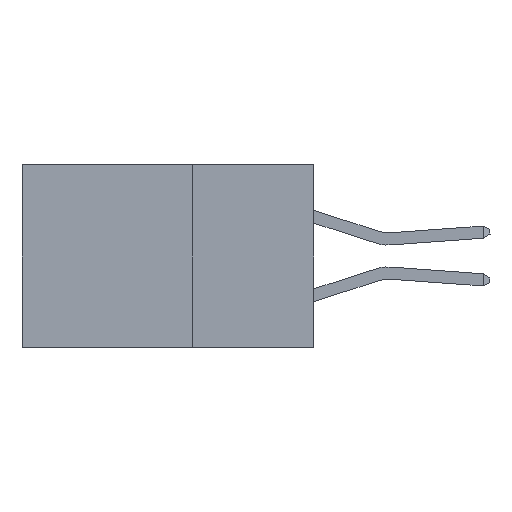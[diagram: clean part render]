
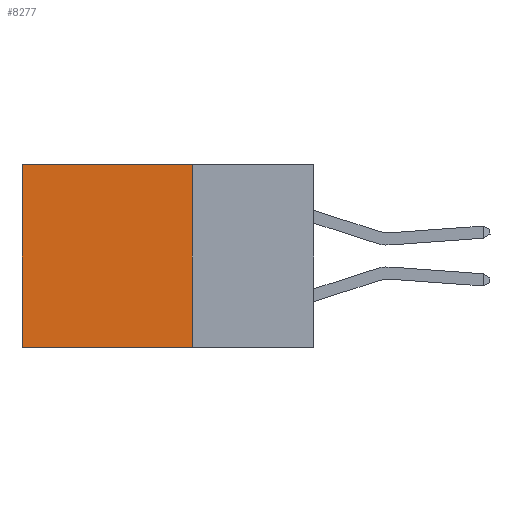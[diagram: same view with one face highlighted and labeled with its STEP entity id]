
A CAD part, left-side view. The second image highlights one B-rep face of the part: STEP entity #8277.
In plain terms, the highlighted planar face has unit normal (-1, 0, 0).
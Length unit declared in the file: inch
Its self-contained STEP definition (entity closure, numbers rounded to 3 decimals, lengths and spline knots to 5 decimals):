
#71 = CARTESIAN_POINT ( 'NONE',  ( 0.2875, 0.25, 0. ) ) ;
#349 = LINE ( 'NONE', #71, #3663 ) ;
#532 = ORIENTED_EDGE ( 'NONE', *, *, #6574, .T. ) ;
#657 = DIRECTION ( 'NONE',  ( 0., 0., -1. ) ) ;
#1223 = ORIENTED_EDGE ( 'NONE', *, *, #1828, .T. ) ;
#1416 = CARTESIAN_POINT ( 'NONE',  ( 0.2875, 0.25, -0.375 ) ) ;
#1828 = EDGE_CURVE ( 'NONE', #12199, #11607, #349, .T. ) ;
#2063 = CARTESIAN_POINT ( 'NONE',  ( 0.2875, 0.6, 0. ) ) ;
#2286 = ORIENTED_EDGE ( 'NONE', *, *, #10214, .F. ) ;
#2362 = CARTESIAN_POINT ( 'NONE',  ( 0.2875, 0.6, -0.375 ) ) ;
#2372 = DIRECTION ( 'NONE',  ( 0., 1., 0. ) ) ;
#2749 = VERTEX_POINT ( 'NONE', #7823 ) ;
#3589 = EDGE_LOOP ( 'NONE', ( #532, #2286, #6079, #1223 ) ) ;
#3663 = VECTOR ( 'NONE', #2372, 39.37008 ) ;
#4012 = LINE ( 'NONE', #10274, #11374 ) ;
#5044 = PLANE ( 'NONE',  #10291 ) ;
#5998 = VECTOR ( 'NONE', #9910, 39.37008 ) ;
#6079 = ORIENTED_EDGE ( 'NONE', *, *, #13675, .F. ) ;
#6574 = EDGE_CURVE ( 'NONE', #11607, #10894, #4012, .T. ) ;
#6714 = LINE ( 'NONE', #1416, #5998 ) ;
#7823 = CARTESIAN_POINT ( 'NONE',  ( 0.2875, 0.25, -0.375 ) ) ;
#8037 = CARTESIAN_POINT ( 'NONE',  ( 0.2875, 0.25, -0.375 ) ) ;
#8277 = ADVANCED_FACE ( 'NONE', ( #12280 ), #5044, .F. ) ;
#9072 = DIRECTION ( 'NONE',  ( 0., 1., 0. ) ) ;
#9275 = CARTESIAN_POINT ( 'NONE',  ( 0.2875, 0.25, -0.375 ) ) ;
#9910 = DIRECTION ( 'NONE',  ( 0., 0., -1. ) ) ;
#10107 = LINE ( 'NONE', #8037, #12419 ) ;
#10214 = EDGE_CURVE ( 'NONE', #2749, #10894, #10107, .T. ) ;
#10274 = CARTESIAN_POINT ( 'NONE',  ( 0.2875, 0.6, -0.375 ) ) ;
#10291 = AXIS2_PLACEMENT_3D ( 'NONE', #9275, #13405, #657 ) ;
#10522 = CARTESIAN_POINT ( 'NONE',  ( 0.2875, 0.25, 0. ) ) ;
#10894 = VERTEX_POINT ( 'NONE', #2362 ) ;
#11249 = DIRECTION ( 'NONE',  ( 0., 0., -1. ) ) ;
#11374 = VECTOR ( 'NONE', #11249, 39.37008 ) ;
#11607 = VERTEX_POINT ( 'NONE', #2063 ) ;
#12199 = VERTEX_POINT ( 'NONE', #10522 ) ;
#12280 = FACE_OUTER_BOUND ( 'NONE', #3589, .T. ) ;
#12419 = VECTOR ( 'NONE', #9072, 39.37008 ) ;
#13405 = DIRECTION ( 'NONE',  ( 1., 0., 0. ) ) ;
#13675 = EDGE_CURVE ( 'NONE', #12199, #2749, #6714, .T. ) ;
